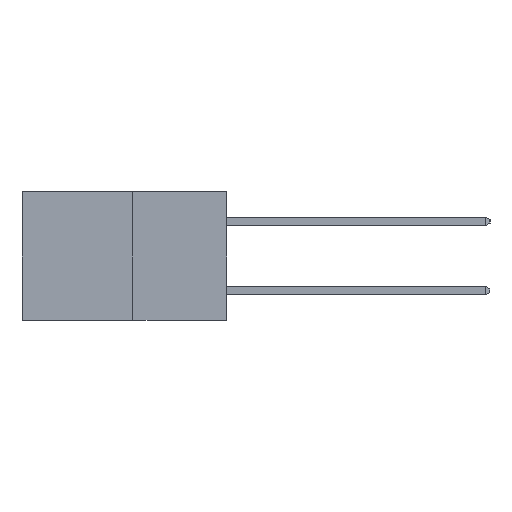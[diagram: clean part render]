
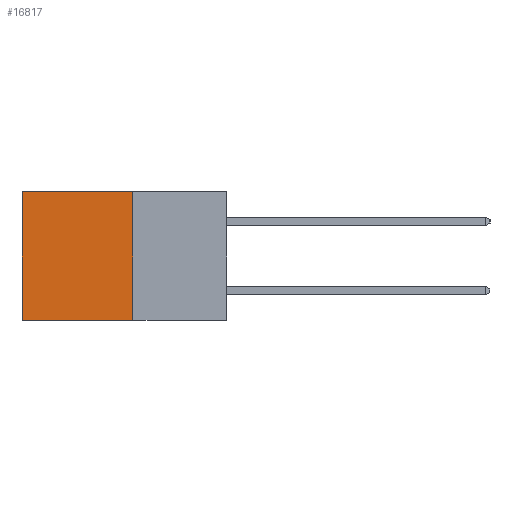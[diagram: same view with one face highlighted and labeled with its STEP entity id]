
A CAD part, left-side view. The second image highlights one B-rep face of the part: STEP entity #16817.
In plain terms, the highlighted planar face has unit normal (-1, 0, 0).
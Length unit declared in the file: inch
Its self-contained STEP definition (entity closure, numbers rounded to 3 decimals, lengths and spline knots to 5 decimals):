
#1164 = VERTEX_POINT ( 'NONE', #16939 ) ;
#1224 = VECTOR ( 'NONE', #13608, 39.37008 ) ;
#2130 = ORIENTED_EDGE ( 'NONE', *, *, #18007, .F. ) ;
#2163 = CARTESIAN_POINT ( 'NONE',  ( 0.277, 0.59, -0.37 ) ) ;
#2395 = VECTOR ( 'NONE', #20648, 39.37008 ) ;
#2572 = CARTESIAN_POINT ( 'NONE',  ( 0.277, 0.27, 0. ) ) ;
#3097 = EDGE_CURVE ( 'NONE', #1164, #27020, #21436, .T. ) ;
#3569 = EDGE_LOOP ( 'NONE', ( #24355, #12379, #2130, #12696 ) ) ;
#3592 = CARTESIAN_POINT ( 'NONE',  ( 0.277, 0.27, -0.37 ) ) ;
#4172 = CARTESIAN_POINT ( 'NONE',  ( 0.277, 0.59, -0.37 ) ) ;
#4487 = CARTESIAN_POINT ( 'NONE',  ( 0.277, 0.27, -0.37 ) ) ;
#5050 = DIRECTION ( 'NONE',  ( 0., 1., 0. ) ) ;
#5953 = VECTOR ( 'NONE', #11606, 39.37008 ) ;
#8172 = LINE ( 'NONE', #3592, #2395 ) ;
#9452 = PLANE ( 'NONE',  #22107 ) ;
#9798 = LINE ( 'NONE', #2572, #21920 ) ;
#10471 = CARTESIAN_POINT ( 'NONE',  ( 0.277, 0.59, 0. ) ) ;
#11606 = DIRECTION ( 'NONE',  ( 0., 0., -1. ) ) ;
#11918 = DIRECTION ( 'NONE',  ( 0., 0., -1. ) ) ;
#12379 = ORIENTED_EDGE ( 'NONE', *, *, #3097, .F. ) ;
#12489 = LINE ( 'NONE', #4172, #5953 ) ;
#12696 = ORIENTED_EDGE ( 'NONE', *, *, #30989, .T. ) ;
#13352 = CARTESIAN_POINT ( 'NONE',  ( 0.277, 0.27, -0.37 ) ) ;
#13608 = DIRECTION ( 'NONE',  ( 0., 1., 0. ) ) ;
#16707 = EDGE_CURVE ( 'NONE', #22690, #27020, #12489, .T. ) ;
#16817 = ADVANCED_FACE ( 'NONE', ( #22296 ), #9452, .F. ) ;
#16939 = CARTESIAN_POINT ( 'NONE',  ( 0.277, 0.27, -0.37 ) ) ;
#18007 = EDGE_CURVE ( 'NONE', #18580, #1164, #8172, .T. ) ;
#18580 = VERTEX_POINT ( 'NONE', #20200 ) ;
#20200 = CARTESIAN_POINT ( 'NONE',  ( 0.277, 0.27, 0. ) ) ;
#20648 = DIRECTION ( 'NONE',  ( 0., 0., -1. ) ) ;
#21436 = LINE ( 'NONE', #13352, #1224 ) ;
#21920 = VECTOR ( 'NONE', #5050, 39.37008 ) ;
#22107 = AXIS2_PLACEMENT_3D ( 'NONE', #4487, #26266, #11918 ) ;
#22296 = FACE_OUTER_BOUND ( 'NONE', #3569, .T. ) ;
#22690 = VERTEX_POINT ( 'NONE', #10471 ) ;
#24355 = ORIENTED_EDGE ( 'NONE', *, *, #16707, .T. ) ;
#26266 = DIRECTION ( 'NONE',  ( 1., 0., 0. ) ) ;
#27020 = VERTEX_POINT ( 'NONE', #2163 ) ;
#30989 = EDGE_CURVE ( 'NONE', #18580, #22690, #9798, .T. ) ;
